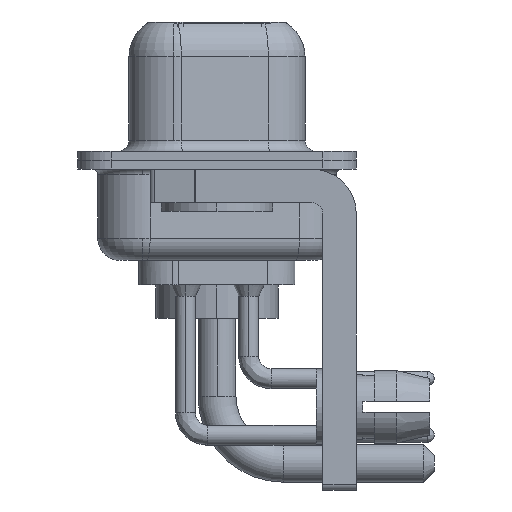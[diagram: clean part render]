
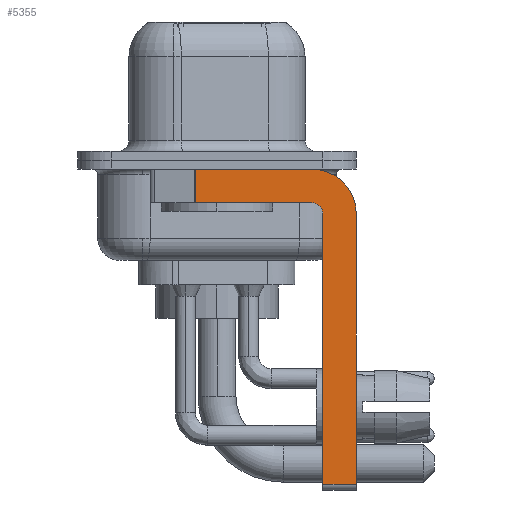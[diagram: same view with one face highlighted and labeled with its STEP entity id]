
A CAD part, left-side view. The second image highlights one B-rep face of the part: STEP entity #5355.
In plain terms, the highlighted planar face has unit normal (-1, 0, 0).
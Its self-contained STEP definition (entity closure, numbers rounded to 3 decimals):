
#79 = VERTEX_POINT ( 'NONE', #5867 ) ;
#510 = FACE_OUTER_BOUND ( 'NONE', #19879, .T. ) ;
#620 = CARTESIAN_POINT ( 'NONE',  ( -2.9, -4.25, -1.9 ) ) ;
#774 = CARTESIAN_POINT ( 'NONE',  ( -2.9, -4.75, -14.8 ) ) ;
#946 = CARTESIAN_POINT ( 'NONE',  ( -2.9, 3., -0.4 ) ) ;
#1408 = CARTESIAN_POINT ( 'NONE',  ( -2.9, -4.75, -14.55 ) ) ;
#1969 = VECTOR ( 'NONE', #4879, 1000. ) ;
#2215 = LINE ( 'NONE', #9564, #11351 ) ;
#2269 = DIRECTION ( 'NONE',  ( 0., -1., 0. ) ) ;
#2565 = VERTEX_POINT ( 'NONE', #15511 ) ;
#2966 = CARTESIAN_POINT ( 'NONE',  ( -2.9, -6.25, -2.4 ) ) ;
#3466 = EDGE_CURVE ( 'NONE', #24176, #20850, #9520, .T. ) ;
#3570 = DIRECTION ( 'NONE',  ( 0., 0., -1. ) ) ;
#4013 = DIRECTION ( 'NONE',  ( -1., 0., 0. ) ) ;
#4233 = AXIS2_PLACEMENT_3D ( 'NONE', #7755, #11183, #3570 ) ;
#4879 = DIRECTION ( 'NONE',  ( 0., 1., 0. ) ) ;
#5049 = VERTEX_POINT ( 'NONE', #8400 ) ;
#5125 = EDGE_CURVE ( 'NONE', #5049, #2565, #10312, .T. ) ;
#5355 = ADVANCED_FACE ( 'NONE', ( #510 ), #21403, .F. ) ;
#5391 = EDGE_CURVE ( 'NONE', #6459, #20850, #6079, .T. ) ;
#5867 = CARTESIAN_POINT ( 'NONE',  ( -2.9, -4.25, -1.9 ) ) ;
#6079 = LINE ( 'NONE', #12138, #17447 ) ;
#6156 = VECTOR ( 'NONE', #16214, 1000. ) ;
#6459 = VERTEX_POINT ( 'NONE', #1408 ) ;
#6642 = ORIENTED_EDGE ( 'NONE', *, *, #12184, .F. ) ;
#7031 = ORIENTED_EDGE ( 'NONE', *, *, #23489, .F. ) ;
#7495 = DIRECTION ( 'NONE',  ( 1., 0., 0. ) ) ;
#7715 = CARTESIAN_POINT ( 'NONE',  ( -2.9, 0.978, -1.9 ) ) ;
#7755 = CARTESIAN_POINT ( 'NONE',  ( -2.9, -4.25, -2.4 ) ) ;
#8219 = DIRECTION ( 'NONE',  ( 0., 0., -1. ) ) ;
#8400 = CARTESIAN_POINT ( 'NONE',  ( -2.9, 0.978, -0.4 ) ) ;
#8925 = EDGE_CURVE ( 'NONE', #2565, #24176, #22841, .T. ) ;
#9520 = LINE ( 'NONE', #17265, #10433 ) ;
#9564 = CARTESIAN_POINT ( 'NONE',  ( -2.9, 0.978, -1.9 ) ) ;
#9858 = CARTESIAN_POINT ( 'NONE',  ( -2.9, -4.25, -2.4 ) ) ;
#10035 = VECTOR ( 'NONE', #20086, 1000. ) ;
#10178 = CARTESIAN_POINT ( 'NONE',  ( -2.9, -4.75, -2.4 ) ) ;
#10312 = LINE ( 'NONE', #946, #10035 ) ;
#10433 = VECTOR ( 'NONE', #24984, 1000. ) ;
#10785 = ORIENTED_EDGE ( 'NONE', *, *, #21078, .T. ) ;
#11183 = DIRECTION ( 'NONE',  ( 1., 0., 0. ) ) ;
#11351 = VECTOR ( 'NONE', #16240, 1000. ) ;
#12138 = CARTESIAN_POINT ( 'NONE',  ( -2.9, -4.25, -14.55 ) ) ;
#12184 = EDGE_CURVE ( 'NONE', #6459, #21036, #18126, .T. ) ;
#12247 = ORIENTED_EDGE ( 'NONE', *, *, #3466, .F. ) ;
#12962 = AXIS2_PLACEMENT_3D ( 'NONE', #23415, #7495, #8219 ) ;
#13093 = CIRCLE ( 'NONE', #13923, 0.5 ) ;
#13923 = AXIS2_PLACEMENT_3D ( 'NONE', #9858, #4013, #20003 ) ;
#15511 = CARTESIAN_POINT ( 'NONE',  ( -2.9, -4.25, -0.4 ) ) ;
#16214 = DIRECTION ( 'NONE',  ( 0., 0., 1. ) ) ;
#16240 = DIRECTION ( 'NONE',  ( 0., 0., -1. ) ) ;
#16838 = ORIENTED_EDGE ( 'NONE', *, *, #17527, .F. ) ;
#17265 = CARTESIAN_POINT ( 'NONE',  ( -2.9, -6.25, -2.4 ) ) ;
#17447 = VECTOR ( 'NONE', #2269, 1000. ) ;
#17527 = EDGE_CURVE ( 'NONE', #79, #21446, #20125, .T. ) ;
#18126 = LINE ( 'NONE', #774, #6156 ) ;
#18477 = CARTESIAN_POINT ( 'NONE',  ( -2.9, -6.25, -14.55 ) ) ;
#19879 = EDGE_LOOP ( 'NONE', ( #21518, #10785, #16838, #7031, #6642, #21844, #12247, #21547 ) ) ;
#20003 = DIRECTION ( 'NONE',  ( 0., 0., 1. ) ) ;
#20086 = DIRECTION ( 'NONE',  ( 0., -1., 0. ) ) ;
#20125 = LINE ( 'NONE', #620, #1969 ) ;
#20850 = VERTEX_POINT ( 'NONE', #18477 ) ;
#21036 = VERTEX_POINT ( 'NONE', #10178 ) ;
#21078 = EDGE_CURVE ( 'NONE', #5049, #21446, #2215, .T. ) ;
#21403 = PLANE ( 'NONE',  #12962 ) ;
#21446 = VERTEX_POINT ( 'NONE', #7715 ) ;
#21518 = ORIENTED_EDGE ( 'NONE', *, *, #5125, .F. ) ;
#21547 = ORIENTED_EDGE ( 'NONE', *, *, #8925, .F. ) ;
#21844 = ORIENTED_EDGE ( 'NONE', *, *, #5391, .T. ) ;
#22841 = CIRCLE ( 'NONE', #4233, 2. ) ;
#23415 = CARTESIAN_POINT ( 'NONE',  ( -2.9, -4.25, -2.4 ) ) ;
#23489 = EDGE_CURVE ( 'NONE', #21036, #79, #13093, .T. ) ;
#24176 = VERTEX_POINT ( 'NONE', #2966 ) ;
#24984 = DIRECTION ( 'NONE',  ( 0., 0., -1. ) ) ;
